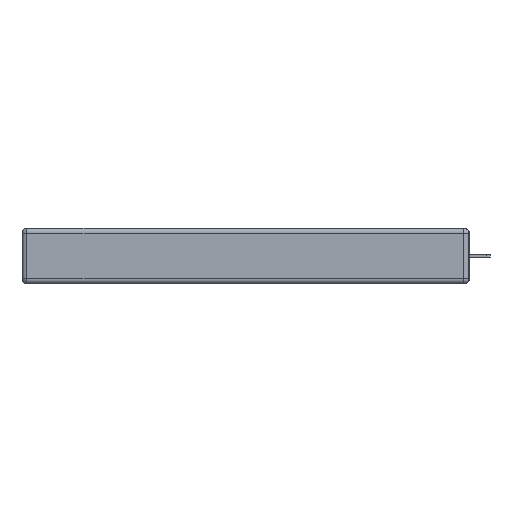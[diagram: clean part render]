
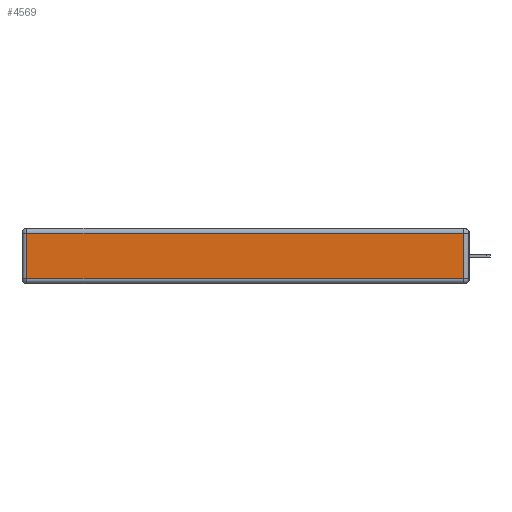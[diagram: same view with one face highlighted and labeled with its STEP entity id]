
A CAD part, left-side view. The second image highlights one B-rep face of the part: STEP entity #4569.
In plain terms, the highlighted planar face has unit normal (-1, 0, 0).
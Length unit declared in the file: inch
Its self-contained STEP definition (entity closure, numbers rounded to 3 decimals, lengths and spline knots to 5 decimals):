
#277 = CARTESIAN_POINT ( 'NONE',  ( 0., 0.03, -0.03 ) ) ;
#1272 = VERTEX_POINT ( 'NONE', #10343 ) ;
#1367 = CARTESIAN_POINT ( 'NONE',  ( 0., 2.72, -0.343 ) ) ;
#1472 = DIRECTION ( 'NONE',  ( 0., 0., -1. ) ) ;
#2904 = CARTESIAN_POINT ( 'NONE',  ( 0., 0.03, -0.343 ) ) ;
#3270 = VERTEX_POINT ( 'NONE', #15908 ) ;
#4343 = CARTESIAN_POINT ( 'NONE',  ( 0., 0., -0.343 ) ) ;
#4350 = LINE ( 'NONE', #21126, #19745 ) ;
#4517 = AXIS2_PLACEMENT_3D ( 'NONE', #4343, #16048, #16159 ) ;
#4569 = ADVANCED_FACE ( 'NONE', ( #21445 ), #9289, .T. ) ;
#5039 = ORIENTED_EDGE ( 'NONE', *, *, #16382, .T. ) ;
#6949 = ORIENTED_EDGE ( 'NONE', *, *, #19628, .T. ) ;
#7147 = VECTOR ( 'NONE', #21108, 39.37008 ) ;
#8046 = EDGE_CURVE ( 'NONE', #21381, #19092, #4350, .T. ) ;
#9289 = PLANE ( 'NONE',  #4517 ) ;
#10063 = VECTOR ( 'NONE', #13781, 39.37008 ) ;
#10343 = CARTESIAN_POINT ( 'NONE',  ( 0., 2.72, -0.313 ) ) ;
#10963 = EDGE_CURVE ( 'NONE', #3270, #21381, #18008, .T. ) ;
#13781 = DIRECTION ( 'NONE',  ( 0., -1., 0. ) ) ;
#14752 = ORIENTED_EDGE ( 'NONE', *, *, #10963, .T. ) ;
#15701 = EDGE_LOOP ( 'NONE', ( #6949, #14752, #21670, #5039 ) ) ;
#15908 = CARTESIAN_POINT ( 'NONE',  ( 0., 0.03, -0.313 ) ) ;
#16048 = DIRECTION ( 'NONE',  ( -1., 0., 0. ) ) ;
#16100 = VECTOR ( 'NONE', #1472, 39.37008 ) ;
#16159 = DIRECTION ( 'NONE',  ( 0., 0., 1. ) ) ;
#16382 = EDGE_CURVE ( 'NONE', #19092, #1272, #16594, .T. ) ;
#16594 = LINE ( 'NONE', #1367, #16100 ) ;
#18008 = LINE ( 'NONE', #2904, #7147 ) ;
#18403 = LINE ( 'NONE', #18726, #10063 ) ;
#18726 = CARTESIAN_POINT ( 'NONE',  ( 0., 0., -0.313 ) ) ;
#19092 = VERTEX_POINT ( 'NONE', #19235 ) ;
#19235 = CARTESIAN_POINT ( 'NONE',  ( 0., 2.72, -0.03 ) ) ;
#19480 = DIRECTION ( 'NONE',  ( 0., 1., 0. ) ) ;
#19628 = EDGE_CURVE ( 'NONE', #1272, #3270, #18403, .T. ) ;
#19745 = VECTOR ( 'NONE', #19480, 39.37008 ) ;
#21108 = DIRECTION ( 'NONE',  ( 0., 0., 1. ) ) ;
#21126 = CARTESIAN_POINT ( 'NONE',  ( 0., 2.75, -0.03 ) ) ;
#21381 = VERTEX_POINT ( 'NONE', #277 ) ;
#21445 = FACE_OUTER_BOUND ( 'NONE', #15701, .T. ) ;
#21670 = ORIENTED_EDGE ( 'NONE', *, *, #8046, .T. ) ;
